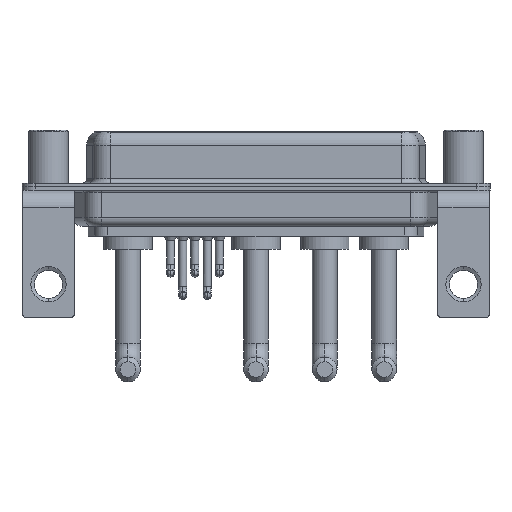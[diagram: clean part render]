
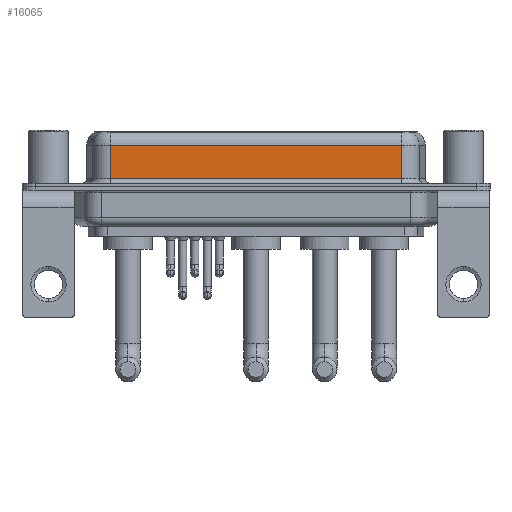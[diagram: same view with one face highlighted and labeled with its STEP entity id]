
A CAD part, front view. The second image highlights one B-rep face of the part: STEP entity #16065.
In plain terms, the highlighted planar face has unit normal (0, -1, 0).
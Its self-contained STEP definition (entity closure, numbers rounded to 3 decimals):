
#2 = VECTOR ( 'NONE', #379, 1000. ) ;
#20 = CARTESIAN_POINT ( 'NONE',  ( 40.037, -3.95, 4.65 ) ) ;
#379 = DIRECTION ( 'NONE',  ( 0., 0., -1. ) ) ;
#573 = ORIENTED_EDGE ( 'NONE', *, *, #16897, .T. ) ;
#896 = AXIS2_PLACEMENT_3D ( 'NONE', #17468, #8450, #16058 ) ;
#1394 = LINE ( 'NONE', #2996, #5458 ) ;
#2306 = CARTESIAN_POINT ( 'NONE',  ( 40.037, -3.95, 4.65 ) ) ;
#2934 = CARTESIAN_POINT ( 'NONE',  ( 40.037, -3.95, 0.9 ) ) ;
#2996 = CARTESIAN_POINT ( 'NONE',  ( 40.037, -3.95, 6.4 ) ) ;
#3104 = ORIENTED_EDGE ( 'NONE', *, *, #18520, .F. ) ;
#5023 = LINE ( 'NONE', #14633, #6409 ) ;
#5187 = EDGE_CURVE ( 'NONE', #15819, #16300, #5023, .T. ) ;
#5458 = VECTOR ( 'NONE', #19421, 1000. ) ;
#5472 = PLANE ( 'NONE',  #896 ) ;
#5870 = CARTESIAN_POINT ( 'NONE',  ( 7.013, -3.95, 0.9 ) ) ;
#6409 = VECTOR ( 'NONE', #17528, 1000. ) ;
#6607 = EDGE_CURVE ( 'NONE', #10603, #15819, #15382, .T. ) ;
#6825 = DIRECTION ( 'NONE',  ( -1., 0., 0. ) ) ;
#6901 = CARTESIAN_POINT ( 'NONE',  ( 7.013, -3.95, 4.65 ) ) ;
#7016 = LINE ( 'NONE', #2306, #13328 ) ;
#8450 = DIRECTION ( 'NONE',  ( 0., 1., 0. ) ) ;
#8708 = EDGE_LOOP ( 'NONE', ( #3104, #573, #19327, #18657 ) ) ;
#10603 = VERTEX_POINT ( 'NONE', #6901 ) ;
#13328 = VECTOR ( 'NONE', #6825, 1000. ) ;
#14090 = CARTESIAN_POINT ( 'NONE',  ( 7.013, -3.95, 6.4 ) ) ;
#14633 = CARTESIAN_POINT ( 'NONE',  ( 40.037, -3.95, 0.9 ) ) ;
#15042 = VERTEX_POINT ( 'NONE', #20 ) ;
#15382 = LINE ( 'NONE', #14090, #2 ) ;
#15819 = VERTEX_POINT ( 'NONE', #5870 ) ;
#16058 = DIRECTION ( 'NONE',  ( 0., 0., 1. ) ) ;
#16065 = ADVANCED_FACE ( 'NONE', ( #17656 ), #5472, .F. ) ;
#16300 = VERTEX_POINT ( 'NONE', #2934 ) ;
#16897 = EDGE_CURVE ( 'NONE', #15042, #10603, #7016, .T. ) ;
#17468 = CARTESIAN_POINT ( 'NONE',  ( 40.037, -3.95, 6.4 ) ) ;
#17528 = DIRECTION ( 'NONE',  ( 1., 0., 0. ) ) ;
#17656 = FACE_OUTER_BOUND ( 'NONE', #8708, .T. ) ;
#18520 = EDGE_CURVE ( 'NONE', #15042, #16300, #1394, .T. ) ;
#18657 = ORIENTED_EDGE ( 'NONE', *, *, #5187, .T. ) ;
#19327 = ORIENTED_EDGE ( 'NONE', *, *, #6607, .T. ) ;
#19421 = DIRECTION ( 'NONE',  ( 0., 0., -1. ) ) ;
